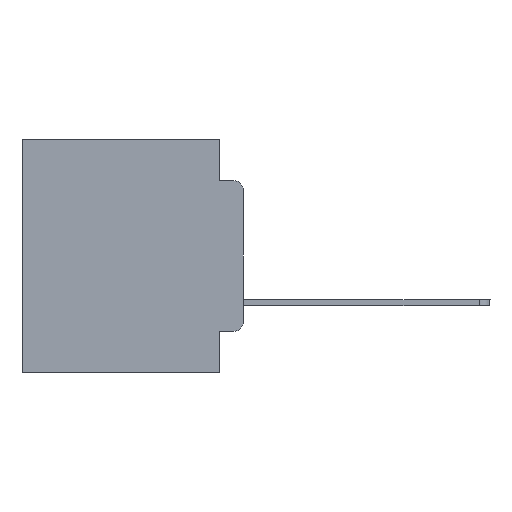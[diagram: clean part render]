
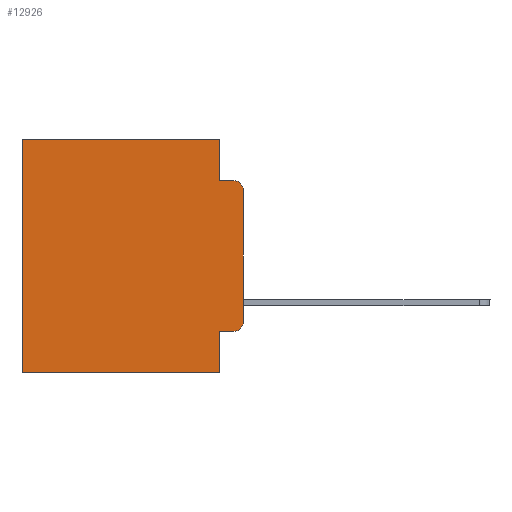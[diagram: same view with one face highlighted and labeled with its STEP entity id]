
A CAD part, left-side view. The second image highlights one B-rep face of the part: STEP entity #12926.
In plain terms, the highlighted planar face has unit normal (-1, 0, 0).
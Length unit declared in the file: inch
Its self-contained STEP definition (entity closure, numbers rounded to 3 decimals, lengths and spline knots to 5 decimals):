
#29 = EDGE_LOOP ( 'NONE', ( #5362, #8195, #19411, #12710, #12299, #17514, #8535, #16314, #21516, #11018 ) ) ;
#169 = DIRECTION ( 'NONE',  ( 0., 0., -1. ) ) ;
#271 = EDGE_CURVE ( 'NONE', #19293, #12465, #17619, .T. ) ;
#851 = EDGE_CURVE ( 'NONE', #22566, #24580, #22481, .T. ) ;
#902 = CARTESIAN_POINT ( 'NONE',  ( 0.298, 0., 0. ) ) ;
#1430 = DIRECTION ( 'NONE',  ( -1., 0., 0. ) ) ;
#1496 = LINE ( 'NONE', #22550, #20904 ) ;
#1574 = VECTOR ( 'NONE', #7755, 39.37008 ) ;
#1686 = CARTESIAN_POINT ( 'NONE',  ( 0.298, 0.051, 0. ) ) ;
#1929 = DIRECTION ( 'NONE',  ( 0., 0., -1. ) ) ;
#2319 = EDGE_CURVE ( 'NONE', #14523, #10170, #6976, .T. ) ;
#2468 = VECTOR ( 'NONE', #169, 39.37008 ) ;
#2676 = CARTESIAN_POINT ( 'NONE',  ( 0.298, 0., -0.3915 ) ) ;
#3066 = FACE_OUTER_BOUND ( 'NONE', #29, .T. ) ;
#3348 = VERTEX_POINT ( 'NONE', #15711 ) ;
#3369 = EDGE_CURVE ( 'NONE', #20157, #19293, #6920, .T. ) ;
#3379 = DIRECTION ( 'NONE',  ( 1., 0., 0. ) ) ;
#3535 = CARTESIAN_POINT ( 'NONE',  ( 0.298, 0.02, -0.0885 ) ) ;
#3556 = DIRECTION ( 'NONE',  ( 0., 0., -1. ) ) ;
#5038 = CARTESIAN_POINT ( 'NONE',  ( 0.298, 0.051, 0. ) ) ;
#5148 = CARTESIAN_POINT ( 'NONE',  ( 0.298, 0.473, 0. ) ) ;
#5362 = ORIENTED_EDGE ( 'NONE', *, *, #17938, .F. ) ;
#5975 = CARTESIAN_POINT ( 'NONE',  ( 0.298, 0.473, -0.5 ) ) ;
#6823 = CARTESIAN_POINT ( 'NONE',  ( 0.298, 0.02, -0.4115 ) ) ;
#6920 = LINE ( 'NONE', #25431, #20203 ) ;
#6941 = VERTEX_POINT ( 'NONE', #12144 ) ;
#6970 = DIRECTION ( 'NONE',  ( 0., 1., 0. ) ) ;
#6976 = CIRCLE ( 'NONE', #16468, 0.02 ) ;
#7611 = CARTESIAN_POINT ( 'NONE',  ( 0.298, 0.02, -0.1085 ) ) ;
#7755 = DIRECTION ( 'NONE',  ( 0., 1., 0. ) ) ;
#7844 = VECTOR ( 'NONE', #10736, 39.37008 ) ;
#8049 = EDGE_CURVE ( 'NONE', #3348, #12465, #19428, .T. ) ;
#8195 = ORIENTED_EDGE ( 'NONE', *, *, #2319, .T. ) ;
#8535 = ORIENTED_EDGE ( 'NONE', *, *, #271, .F. ) ;
#9019 = DIRECTION ( 'NONE',  ( 0., 0., -1. ) ) ;
#10170 = VERTEX_POINT ( 'NONE', #3535 ) ;
#10282 = LINE ( 'NONE', #22018, #20146 ) ;
#10736 = DIRECTION ( 'NONE',  ( 0., 0., -1. ) ) ;
#11018 = ORIENTED_EDGE ( 'NONE', *, *, #851, .T. ) ;
#11835 = CARTESIAN_POINT ( 'NONE',  ( 0.298, 0., -0.1085 ) ) ;
#11977 = CARTESIAN_POINT ( 'NONE',  ( 0.298, 0., 0. ) ) ;
#12144 = CARTESIAN_POINT ( 'NONE',  ( 0.298, 0.051, -0.0885 ) ) ;
#12299 = ORIENTED_EDGE ( 'NONE', *, *, #24183, .T. ) ;
#12437 = DIRECTION ( 'NONE',  ( 0., -1., 0. ) ) ;
#12465 = VERTEX_POINT ( 'NONE', #5975 ) ;
#12710 = ORIENTED_EDGE ( 'NONE', *, *, #15460, .F. ) ;
#12926 = ADVANCED_FACE ( 'NONE', ( #3066 ), #23160, .F. ) ;
#13309 = CARTESIAN_POINT ( 'NONE',  ( 0.298, 0., 0. ) ) ;
#13318 = EDGE_CURVE ( 'NONE', #20157, #22566, #1496, .T. ) ;
#14523 = VERTEX_POINT ( 'NONE', #11835 ) ;
#15202 = DIRECTION ( 'NONE',  ( 0., 0., -1. ) ) ;
#15460 = EDGE_CURVE ( 'NONE', #15467, #6941, #22321, .T. ) ;
#15467 = VERTEX_POINT ( 'NONE', #1686 ) ;
#15616 = CARTESIAN_POINT ( 'NONE',  ( 0.298, 0., -0.5 ) ) ;
#15711 = CARTESIAN_POINT ( 'NONE',  ( 0.298, 0.473, 0. ) ) ;
#16269 = AXIS2_PLACEMENT_3D ( 'NONE', #22760, #1430, #15202 ) ;
#16314 = ORIENTED_EDGE ( 'NONE', *, *, #3369, .F. ) ;
#16378 = CARTESIAN_POINT ( 'NONE',  ( 0.298, 0.051, -0.4115 ) ) ;
#16468 = AXIS2_PLACEMENT_3D ( 'NONE', #7611, #17540, #19357 ) ;
#17514 = ORIENTED_EDGE ( 'NONE', *, *, #8049, .T. ) ;
#17540 = DIRECTION ( 'NONE',  ( -1., 0., 0. ) ) ;
#17619 = LINE ( 'NONE', #15616, #1574 ) ;
#17938 = EDGE_CURVE ( 'NONE', #14523, #24580, #24616, .T. ) ;
#19293 = VERTEX_POINT ( 'NONE', #23719 ) ;
#19357 = DIRECTION ( 'NONE',  ( 0., 0., -1. ) ) ;
#19379 = LINE ( 'NONE', #902, #23034 ) ;
#19411 = ORIENTED_EDGE ( 'NONE', *, *, #20734, .F. ) ;
#19428 = LINE ( 'NONE', #5148, #24878 ) ;
#20146 = VECTOR ( 'NONE', #22182, 39.37008 ) ;
#20157 = VERTEX_POINT ( 'NONE', #16378 ) ;
#20203 = VECTOR ( 'NONE', #1929, 39.37008 ) ;
#20733 = AXIS2_PLACEMENT_3D ( 'NONE', #13309, #3379, #3556 ) ;
#20734 = EDGE_CURVE ( 'NONE', #6941, #10170, #10282, .T. ) ;
#20904 = VECTOR ( 'NONE', #12437, 39.37008 ) ;
#21516 = ORIENTED_EDGE ( 'NONE', *, *, #13318, .T. ) ;
#22018 = CARTESIAN_POINT ( 'NONE',  ( 0.298, 0.051, -0.0885 ) ) ;
#22182 = DIRECTION ( 'NONE',  ( 0., -1., 0. ) ) ;
#22321 = LINE ( 'NONE', #5038, #7844 ) ;
#22481 = CIRCLE ( 'NONE', #16269, 0.02 ) ;
#22550 = CARTESIAN_POINT ( 'NONE',  ( 0.298, 0.051, -0.4115 ) ) ;
#22566 = VERTEX_POINT ( 'NONE', #6823 ) ;
#22760 = CARTESIAN_POINT ( 'NONE',  ( 0.298, 0.02, -0.3915 ) ) ;
#23034 = VECTOR ( 'NONE', #6970, 39.37008 ) ;
#23160 = PLANE ( 'NONE',  #20733 ) ;
#23719 = CARTESIAN_POINT ( 'NONE',  ( 0.298, 0.051, -0.5 ) ) ;
#24183 = EDGE_CURVE ( 'NONE', #15467, #3348, #19379, .T. ) ;
#24580 = VERTEX_POINT ( 'NONE', #2676 ) ;
#24616 = LINE ( 'NONE', #11977, #2468 ) ;
#24878 = VECTOR ( 'NONE', #9019, 39.37008 ) ;
#25431 = CARTESIAN_POINT ( 'NONE',  ( 0.298, 0.051, 0. ) ) ;
